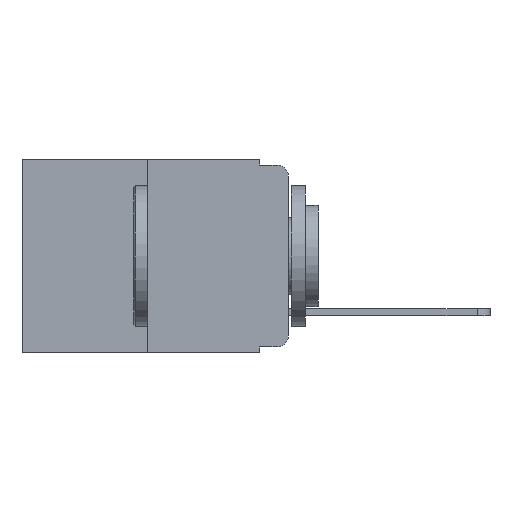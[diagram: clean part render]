
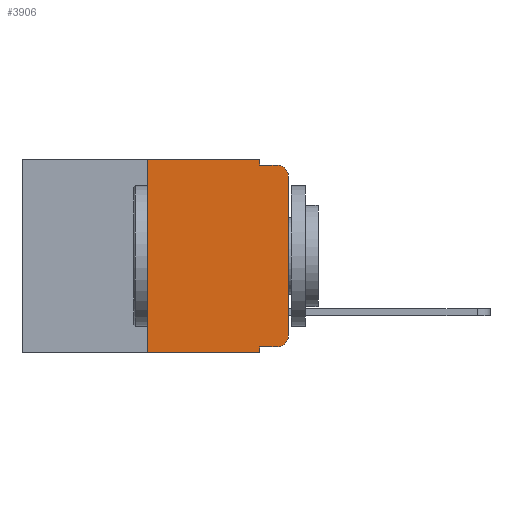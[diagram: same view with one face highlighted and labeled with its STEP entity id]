
A CAD part, left-side view. The second image highlights one B-rep face of the part: STEP entity #3906.
In plain terms, the highlighted planar face has unit normal (-1, 0, 0).
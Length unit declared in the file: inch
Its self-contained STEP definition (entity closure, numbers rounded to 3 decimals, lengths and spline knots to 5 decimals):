
#66 = VECTOR ( 'NONE', #2627, 39.37008 ) ;
#68 = DIRECTION ( 'NONE',  ( 0., -1., 0. ) ) ;
#87 = EDGE_LOOP ( 'NONE', ( #10106, #5623, #8033, #10391, #8304, #10679, #1378, #8879, #11225, #6775 ) ) ;
#348 = CARTESIAN_POINT ( 'NONE',  ( 0., 0.02, -0.333 ) ) ;
#491 = CARTESIAN_POINT ( 'NONE',  ( 0., 0.25, -0.343 ) ) ;
#573 = VERTEX_POINT ( 'NONE', #348 ) ;
#800 = DIRECTION ( 'NONE',  ( 0., -1., 0. ) ) ;
#1047 = VECTOR ( 'NONE', #6022, 39.37008 ) ;
#1098 = DIRECTION ( 'NONE',  ( 0., 0., -1. ) ) ;
#1126 = VERTEX_POINT ( 'NONE', #9516 ) ;
#1319 = LINE ( 'NONE', #4605, #1047 ) ;
#1378 = ORIENTED_EDGE ( 'NONE', *, *, #6453, .T. ) ;
#1748 = EDGE_CURVE ( 'NONE', #573, #9635, #2647, .T. ) ;
#1760 = LINE ( 'NONE', #5230, #7432 ) ;
#2208 = LINE ( 'NONE', #8275, #11691 ) ;
#2420 = FACE_OUTER_BOUND ( 'NONE', #87, .T. ) ;
#2627 = DIRECTION ( 'NONE',  ( 0., -1., 0. ) ) ;
#2647 = CIRCLE ( 'NONE', #3952, 0.02 ) ;
#3097 = EDGE_CURVE ( 'NONE', #1126, #573, #11108, .T. ) ;
#3222 = VERTEX_POINT ( 'NONE', #7453 ) ;
#3315 = CARTESIAN_POINT ( 'NONE',  ( 0., 0.051, -0.333 ) ) ;
#3327 = CARTESIAN_POINT ( 'NONE',  ( 0., 0., 0. ) ) ;
#3649 = DIRECTION ( 'NONE',  ( -1., 0., 0. ) ) ;
#3746 = EDGE_CURVE ( 'NONE', #1126, #5188, #4236, .T. ) ;
#3837 = VERTEX_POINT ( 'NONE', #9436 ) ;
#3855 = CARTESIAN_POINT ( 'NONE',  ( 0., 0.473, -0.343 ) ) ;
#3879 = LINE ( 'NONE', #3855, #6132 ) ;
#3906 = ADVANCED_FACE ( 'NONE', ( #2420 ), #8054, .F. ) ;
#3952 = AXIS2_PLACEMENT_3D ( 'NONE', #6170, #4932, #1098 ) ;
#3975 = LINE ( 'NONE', #3327, #8592 ) ;
#4236 = LINE ( 'NONE', #11158, #11472 ) ;
#4266 = DIRECTION ( 'NONE',  ( 0., 0., 1. ) ) ;
#4359 = AXIS2_PLACEMENT_3D ( 'NONE', #8007, #7852, #7782 ) ;
#4366 = EDGE_CURVE ( 'NONE', #7387, #3222, #1760, .T. ) ;
#4455 = DIRECTION ( 'NONE',  ( 0., -1., 0. ) ) ;
#4605 = CARTESIAN_POINT ( 'NONE',  ( 0., 0.051, 0. ) ) ;
#4807 = LINE ( 'NONE', #9155, #66 ) ;
#4932 = DIRECTION ( 'NONE',  ( -1., 0., 0. ) ) ;
#5002 = EDGE_CURVE ( 'NONE', #11232, #3837, #1319, .T. ) ;
#5188 = VERTEX_POINT ( 'NONE', #5625 ) ;
#5230 = CARTESIAN_POINT ( 'NONE',  ( 0., 0.25, 0. ) ) ;
#5380 = DIRECTION ( 'NONE',  ( 0., 0., 1. ) ) ;
#5496 = CIRCLE ( 'NONE', #10953, 0.02 ) ;
#5623 = ORIENTED_EDGE ( 'NONE', *, *, #6902, .T. ) ;
#5625 = CARTESIAN_POINT ( 'NONE',  ( 0., 0.051, -0.343 ) ) ;
#6022 = DIRECTION ( 'NONE',  ( 0., 0., -1. ) ) ;
#6132 = VECTOR ( 'NONE', #68, 39.37008 ) ;
#6170 = CARTESIAN_POINT ( 'NONE',  ( 0., 0.02, -0.313 ) ) ;
#6301 = EDGE_CURVE ( 'NONE', #3837, #7003, #2208, .T. ) ;
#6351 = VERTEX_POINT ( 'NONE', #7449 ) ;
#6453 = EDGE_CURVE ( 'NONE', #7387, #5188, #3879, .T. ) ;
#6775 = ORIENTED_EDGE ( 'NONE', *, *, #1748, .T. ) ;
#6902 = EDGE_CURVE ( 'NONE', #6351, #7003, #5496, .T. ) ;
#7003 = VERTEX_POINT ( 'NONE', #7479 ) ;
#7387 = VERTEX_POINT ( 'NONE', #491 ) ;
#7432 = VECTOR ( 'NONE', #5380, 39.37008 ) ;
#7449 = CARTESIAN_POINT ( 'NONE',  ( 0., 0., -0.03 ) ) ;
#7453 = CARTESIAN_POINT ( 'NONE',  ( 0., 0.25, 0. ) ) ;
#7479 = CARTESIAN_POINT ( 'NONE',  ( 0., 0.02, -0.01 ) ) ;
#7496 = EDGE_CURVE ( 'NONE', #9635, #6351, #3975, .T. ) ;
#7782 = DIRECTION ( 'NONE',  ( 0., 0., -1. ) ) ;
#7852 = DIRECTION ( 'NONE',  ( 1., 0., 0. ) ) ;
#8007 = CARTESIAN_POINT ( 'NONE',  ( 0., 0.473, 0. ) ) ;
#8033 = ORIENTED_EDGE ( 'NONE', *, *, #6301, .F. ) ;
#8054 = PLANE ( 'NONE',  #4359 ) ;
#8275 = CARTESIAN_POINT ( 'NONE',  ( 0., 0.051, -0.01 ) ) ;
#8304 = ORIENTED_EDGE ( 'NONE', *, *, #10801, .F. ) ;
#8592 = VECTOR ( 'NONE', #4266, 39.37008 ) ;
#8879 = ORIENTED_EDGE ( 'NONE', *, *, #3746, .F. ) ;
#9155 = CARTESIAN_POINT ( 'NONE',  ( 0., 0.473, 0. ) ) ;
#9166 = CARTESIAN_POINT ( 'NONE',  ( 0., 0.02, -0.03 ) ) ;
#9184 = DIRECTION ( 'NONE',  ( 0., 0., -1. ) ) ;
#9436 = CARTESIAN_POINT ( 'NONE',  ( 0., 0.051, -0.01 ) ) ;
#9516 = CARTESIAN_POINT ( 'NONE',  ( 0., 0.051, -0.333 ) ) ;
#9635 = VERTEX_POINT ( 'NONE', #11217 ) ;
#10037 = DIRECTION ( 'NONE',  ( 0., 0., -1. ) ) ;
#10106 = ORIENTED_EDGE ( 'NONE', *, *, #7496, .T. ) ;
#10391 = ORIENTED_EDGE ( 'NONE', *, *, #5002, .F. ) ;
#10663 = CARTESIAN_POINT ( 'NONE',  ( 0., 0.051, 0. ) ) ;
#10679 = ORIENTED_EDGE ( 'NONE', *, *, #4366, .F. ) ;
#10801 = EDGE_CURVE ( 'NONE', #3222, #11232, #4807, .T. ) ;
#10849 = VECTOR ( 'NONE', #4455, 39.37008 ) ;
#10953 = AXIS2_PLACEMENT_3D ( 'NONE', #9166, #3649, #10037 ) ;
#11108 = LINE ( 'NONE', #3315, #10849 ) ;
#11158 = CARTESIAN_POINT ( 'NONE',  ( 0., 0.051, 0. ) ) ;
#11217 = CARTESIAN_POINT ( 'NONE',  ( 0., 0., -0.313 ) ) ;
#11225 = ORIENTED_EDGE ( 'NONE', *, *, #3097, .T. ) ;
#11232 = VERTEX_POINT ( 'NONE', #10663 ) ;
#11472 = VECTOR ( 'NONE', #9184, 39.37008 ) ;
#11691 = VECTOR ( 'NONE', #800, 39.37008 ) ;
